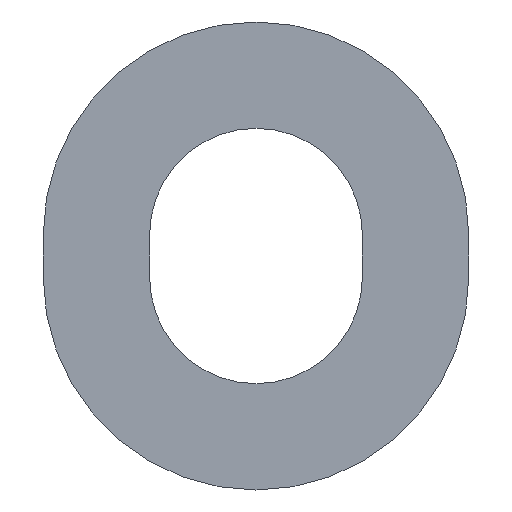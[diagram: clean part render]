
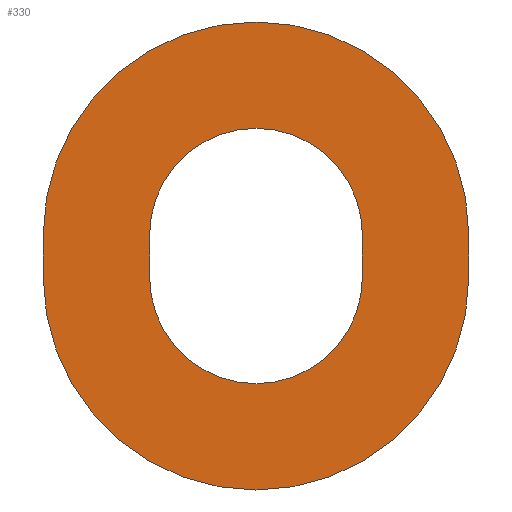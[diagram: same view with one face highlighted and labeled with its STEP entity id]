
A CAD part, front view. The second image highlights one B-rep face of the part: STEP entity #330.
In plain terms, the highlighted planar face has unit normal (0, -1, 0).
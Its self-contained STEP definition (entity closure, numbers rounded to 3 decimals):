
#4 = DIRECTION ( 'NONE',  ( 0., 1., 0. ) ) ;
#8 = EDGE_CURVE ( 'NONE', #209, #437, #159, .T. ) ;
#9 = DIRECTION ( 'NONE',  ( 0., 1., 0. ) ) ;
#11 = CARTESIAN_POINT ( 'NONE',  ( 2.5, 0., -1. ) ) ;
#16 = FACE_BOUND ( 'NONE', #417, .T. ) ;
#20 = CARTESIAN_POINT ( 'NONE',  ( 0., 0., -1. ) ) ;
#21 = CARTESIAN_POINT ( 'NONE',  ( 5., 0., 0. ) ) ;
#22 = CARTESIAN_POINT ( 'NONE',  ( -5., 0., -1. ) ) ;
#30 = CARTESIAN_POINT ( 'NONE',  ( -2.5, 0., 0. ) ) ;
#32 = CIRCLE ( 'NONE', #362, 5. ) ;
#38 = EDGE_CURVE ( 'NONE', #389, #409, #160, .T. ) ;
#47 = CIRCLE ( 'NONE', #377, 2.5 ) ;
#48 = CARTESIAN_POINT ( 'NONE',  ( -5., 0., 0. ) ) ;
#54 = CARTESIAN_POINT ( 'NONE',  ( 0., 0., 0. ) ) ;
#55 = VERTEX_POINT ( 'NONE', #48 ) ;
#70 = DIRECTION ( 'NONE',  ( 0., 0., 1. ) ) ;
#81 = EDGE_CURVE ( 'NONE', #101, #55, #151, .T. ) ;
#87 = CARTESIAN_POINT ( 'NONE',  ( 0., 0., -3.5 ) ) ;
#94 = FACE_OUTER_BOUND ( 'NONE', #446, .T. ) ;
#101 = VERTEX_POINT ( 'NONE', #22 ) ;
#106 = DIRECTION ( 'NONE',  ( 0., 1., 0. ) ) ;
#122 = DIRECTION ( 'NONE',  ( 0., 0., 1. ) ) ;
#128 = VECTOR ( 'NONE', #246, 1000. ) ;
#129 = CIRCLE ( 'NONE', #402, 5. ) ;
#130 = CIRCLE ( 'NONE', #404, 2.5 ) ;
#133 = VECTOR ( 'NONE', #247, 1000. ) ;
#141 = CIRCLE ( 'NONE', #401, 2.5 ) ;
#143 = LINE ( 'NONE', #21, #128 ) ;
#146 = VECTOR ( 'NONE', #156, 1000. ) ;
#149 = EDGE_CURVE ( 'NONE', #55, #329, #154, .T. ) ;
#151 = LINE ( 'NONE', #449, #133 ) ;
#154 = CIRCLE ( 'NONE', #405, 5. ) ;
#155 = VECTOR ( 'NONE', #300, 1000. ) ;
#156 = DIRECTION ( 'NONE',  ( 0., 0., -1. ) ) ;
#159 = LINE ( 'NONE', #326, #155 ) ;
#160 = LINE ( 'NONE', #239, #146 ) ;
#172 = PLANE ( 'NONE',  #395 ) ;
#177 = DIRECTION ( 'NONE',  ( 0., 1., 0. ) ) ;
#183 = DIRECTION ( 'NONE',  ( 0., 1., 0. ) ) ;
#192 = EDGE_CURVE ( 'NONE', #437, #389, #130, .T. ) ;
#196 = CARTESIAN_POINT ( 'NONE',  ( 0., 0., -1. ) ) ;
#200 = CARTESIAN_POINT ( 'NONE',  ( 0., 0., 0. ) ) ;
#201 = EDGE_CURVE ( 'NONE', #329, #407, #143, .T. ) ;
#204 = DIRECTION ( 'NONE',  ( 0., 0., 1. ) ) ;
#209 = VERTEX_POINT ( 'NONE', #344 ) ;
#213 = EDGE_CURVE ( 'NONE', #407, #325, #129, .T. ) ;
#218 = EDGE_CURVE ( 'NONE', #354, #209, #141, .T. ) ;
#222 = ORIENTED_EDGE ( 'NONE', *, *, #149, .F. ) ;
#223 = ORIENTED_EDGE ( 'NONE', *, *, #81, .F. ) ;
#224 = ORIENTED_EDGE ( 'NONE', *, *, #414, .F. ) ;
#228 = DIRECTION ( 'NONE',  ( 0., 0., 1. ) ) ;
#233 = ORIENTED_EDGE ( 'NONE', *, *, #213, .F. ) ;
#235 = ORIENTED_EDGE ( 'NONE', *, *, #201, .F. ) ;
#236 = ORIENTED_EDGE ( 'NONE', *, *, #192, .T. ) ;
#237 = ORIENTED_EDGE ( 'NONE', *, *, #38, .T. ) ;
#239 = CARTESIAN_POINT ( 'NONE',  ( 2.5, 0., 0. ) ) ;
#240 = ORIENTED_EDGE ( 'NONE', *, *, #406, .T. ) ;
#241 = ORIENTED_EDGE ( 'NONE', *, *, #218, .T. ) ;
#243 = ORIENTED_EDGE ( 'NONE', *, *, #8, .T. ) ;
#245 = DIRECTION ( 'NONE',  ( 0., 1., 0. ) ) ;
#246 = DIRECTION ( 'NONE',  ( 0., 0., -1. ) ) ;
#247 = DIRECTION ( 'NONE',  ( 0., 0., 1. ) ) ;
#258 = CARTESIAN_POINT ( 'NONE',  ( 2.5, 0., 0. ) ) ;
#287 = CARTESIAN_POINT ( 'NONE',  ( 0., 0., -6. ) ) ;
#288 = CARTESIAN_POINT ( 'NONE',  ( 0., 0., -1. ) ) ;
#300 = DIRECTION ( 'NONE',  ( 0., 0., 1. ) ) ;
#305 = DIRECTION ( 'NONE',  ( 0., 1., 0. ) ) ;
#320 = DIRECTION ( 'NONE',  ( 0., 0., 1. ) ) ;
#325 = VERTEX_POINT ( 'NONE', #287 ) ;
#326 = CARTESIAN_POINT ( 'NONE',  ( -2.5, 0., 0. ) ) ;
#329 = VERTEX_POINT ( 'NONE', #447 ) ;
#330 = ADVANCED_FACE ( 'NONE', ( #94, #16 ), #172, .F. ) ;
#344 = CARTESIAN_POINT ( 'NONE',  ( -2.5, 0., -1. ) ) ;
#354 = VERTEX_POINT ( 'NONE', #87 ) ;
#362 = AXIS2_PLACEMENT_3D ( 'NONE', #288, #106, #320 ) ;
#375 = DIRECTION ( 'NONE',  ( 0., 0., 1. ) ) ;
#377 = AXIS2_PLACEMENT_3D ( 'NONE', #391, #177, #204 ) ;
#389 = VERTEX_POINT ( 'NONE', #258 ) ;
#391 = CARTESIAN_POINT ( 'NONE',  ( 0., 0., -1. ) ) ;
#395 = AXIS2_PLACEMENT_3D ( 'NONE', #200, #9, #70 ) ;
#401 = AXIS2_PLACEMENT_3D ( 'NONE', #196, #4, #228 ) ;
#402 = AXIS2_PLACEMENT_3D ( 'NONE', #20, #245, #375 ) ;
#403 = CARTESIAN_POINT ( 'NONE',  ( 0., 0., 0. ) ) ;
#404 = AXIS2_PLACEMENT_3D ( 'NONE', #54, #305, #122 ) ;
#405 = AXIS2_PLACEMENT_3D ( 'NONE', #403, #183, #448 ) ;
#406 = EDGE_CURVE ( 'NONE', #409, #354, #47, .T. ) ;
#407 = VERTEX_POINT ( 'NONE', #441 ) ;
#409 = VERTEX_POINT ( 'NONE', #11 ) ;
#414 = EDGE_CURVE ( 'NONE', #325, #101, #32, .T. ) ;
#417 = EDGE_LOOP ( 'NONE', ( #236, #237, #240, #241, #243 ) ) ;
#437 = VERTEX_POINT ( 'NONE', #30 ) ;
#441 = CARTESIAN_POINT ( 'NONE',  ( 5., 0., -1. ) ) ;
#446 = EDGE_LOOP ( 'NONE', ( #222, #223, #224, #233, #235 ) ) ;
#447 = CARTESIAN_POINT ( 'NONE',  ( 5., 0., 0. ) ) ;
#448 = DIRECTION ( 'NONE',  ( 0., 0., 1. ) ) ;
#449 = CARTESIAN_POINT ( 'NONE',  ( -5., 0., 0. ) ) ;
